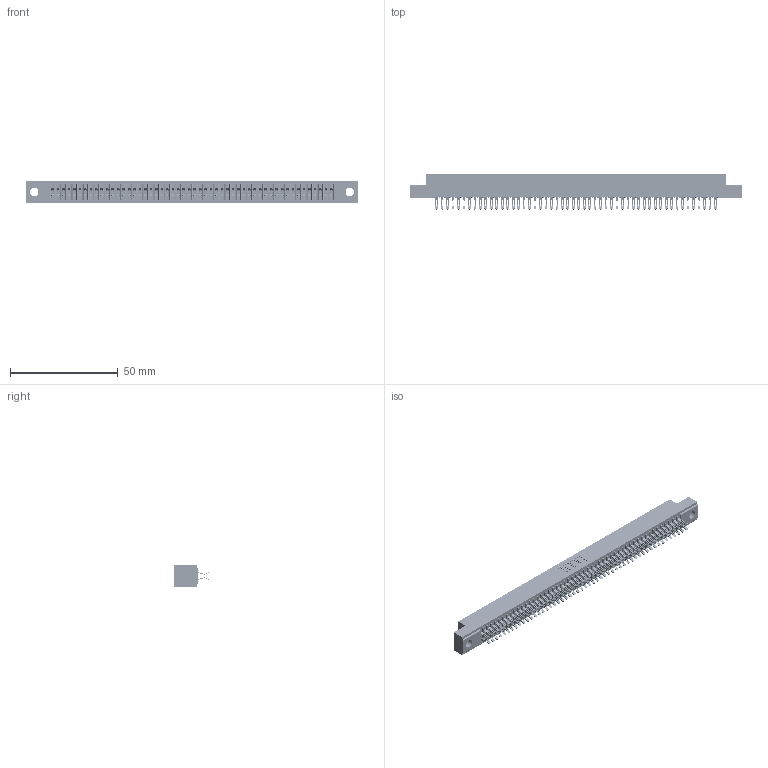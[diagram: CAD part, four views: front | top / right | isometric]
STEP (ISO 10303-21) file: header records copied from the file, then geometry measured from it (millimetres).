
FILE_DESCRIPTION (( 'STEP AP203' ), '1' );
FILE_NAME ('341-104-555-204.STEP', '2018-08-08T11:38:37', ( '' ), ( '' ), 'SwSTEP 2.0', 'SolidWorks 2016', '' );
FILE_SCHEMA (( 'CONFIG_CONTROL_DESIGN' ));
Length unit declared in the file: inch
Products named in the file (3): 341-292-001_341-292-155; 341-104-555-204; 341 Part_.156 (3.96) Dia Mounting Holes
Assembly tree (105 placements, depth 2):
  341-104-555-204
    341 Part_.156 (3.96) Dia Mounting Holes
    341-292-001_341-292-155  x104
Bounding box: 154.31 x 16.31 x 10.16 mm (x, y, z)
Volume: 11429.7 mm3; surface area: 21340 mm2
Topology: 105 solids, 105 shells, 8242 faces, 24636 edges, 16038 vertices
Faces by surface type: plane 4450, cylinder 3584, sphere 106, torus 102
Entity records: 62487 total; most frequent: CARTESIAN_POINT 10408, ORIENTED_EDGE 10332, DIRECTION 10076, EDGE_CURVE 5166, VECTOR 4176, LINE 4176, VERTEX_POINT 3266, AXIS2_PLACEMENT_3D 2950
